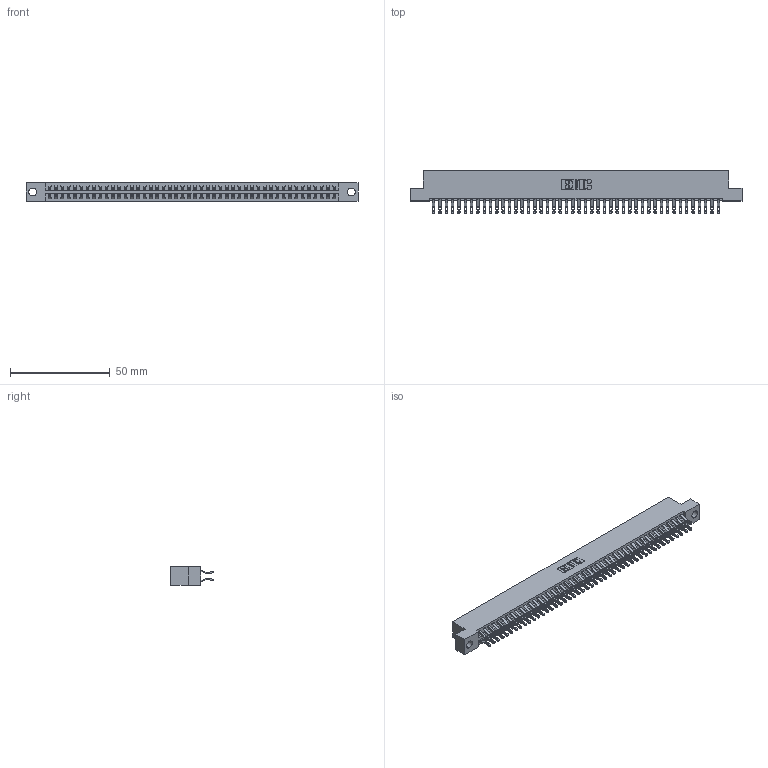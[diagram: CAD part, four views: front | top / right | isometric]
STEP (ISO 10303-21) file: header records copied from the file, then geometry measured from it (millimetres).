
FILE_DESCRIPTION (( 'STEP AP203' ), '1' );
FILE_NAME ('396-092-555-204.STEP', '2019-10-31T02:49:22', ( '' ), ( '' ), 'SwSTEP 2.0', 'SolidWorks 2016', '' );
FILE_SCHEMA (( 'CONFIG_CONTROL_DESIGN' ));
Length unit declared in the file: inch
Products named in the file (3): 345-292-001_555 Tail; 346 Part_Flush Mounting Lugs - 0.156 Dia-TH; 396-092-555-204
Assembly tree (93 placements, depth 2):
  396-092-555-204
    346 Part_Flush Mounting Lugs - 0.156 Dia-TH
    345-292-001_555 Tail  x92
Bounding box: 166.62 x 21.46 x 9.4 mm (x, y, z)
Volume: 16458 mm3; surface area: 23450 mm2
Topology: 93 solids, 93 shells, 5458 faces, 17165 edges, 11442 vertices
Faces by surface type: plane 3112, cylinder 2346
Entity records: 29811 total; most frequent: CARTESIAN_POINT 4942, ORIENTED_EDGE 4846, DIRECTION 4375, EDGE_CURVE 2423, VECTOR 2087, LINE 2087, VERTEX_POINT 1614, AXIS2_PLACEMENT_3D 1144
